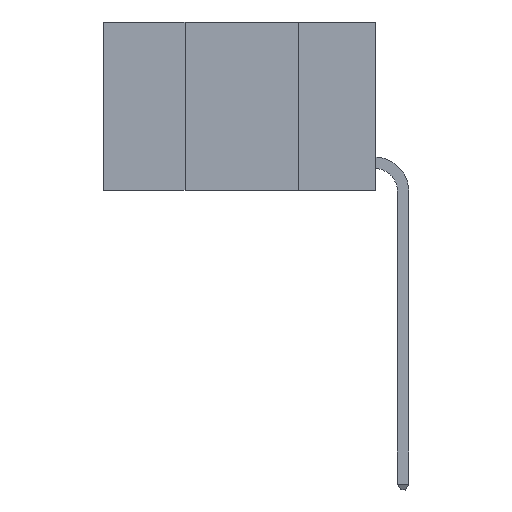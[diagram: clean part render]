
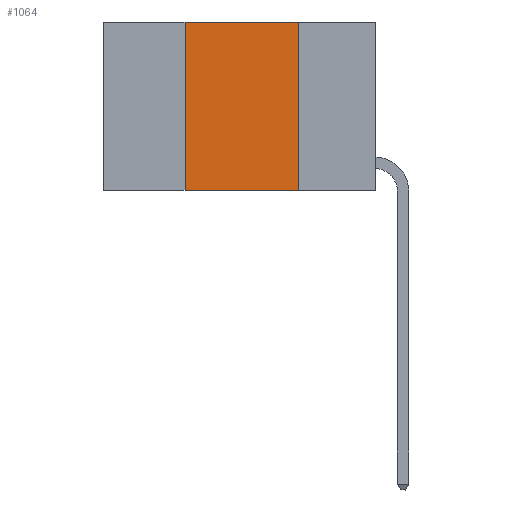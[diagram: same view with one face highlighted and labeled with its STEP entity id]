
A CAD part, left-side view. The second image highlights one B-rep face of the part: STEP entity #1064.
In plain terms, the highlighted planar face has unit normal (-1, 0, 0).
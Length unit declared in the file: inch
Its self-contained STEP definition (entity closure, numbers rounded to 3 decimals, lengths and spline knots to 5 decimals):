
#265 = VERTEX_POINT ( 'NONE', #9439 ) ;
#403 = DIRECTION ( 'NONE',  ( 1., 0., 0. ) ) ;
#446 = LINE ( 'NONE', #10689, #5363 ) ;
#1064 = ADVANCED_FACE ( 'NONE', ( #3475 ), #9762, .F. ) ;
#1499 = EDGE_CURVE ( 'NONE', #8448, #265, #7841, .T. ) ;
#1986 = CARTESIAN_POINT ( 'NONE',  ( 0., 0.42, -0.37 ) ) ;
#2323 = VECTOR ( 'NONE', #11341, 39.37008 ) ;
#2558 = VECTOR ( 'NONE', #10850, 39.37008 ) ;
#2686 = LINE ( 'NONE', #2783, #2323 ) ;
#2783 = CARTESIAN_POINT ( 'NONE',  ( 0., 0.6, 0. ) ) ;
#3475 = FACE_OUTER_BOUND ( 'NONE', #5298, .T. ) ;
#3616 = VECTOR ( 'NONE', #5519, 39.37008 ) ;
#5298 = EDGE_LOOP ( 'NONE', ( #11200, #9071, #10751, #11490 ) ) ;
#5363 = VECTOR ( 'NONE', #6073, 39.37008 ) ;
#5519 = DIRECTION ( 'NONE',  ( 0., 0., 1. ) ) ;
#6073 = DIRECTION ( 'NONE',  ( 0., -1., 0. ) ) ;
#6665 = CARTESIAN_POINT ( 'NONE',  ( 0., 0.42, 0. ) ) ;
#7224 = VERTEX_POINT ( 'NONE', #10201 ) ;
#7841 = LINE ( 'NONE', #6665, #3616 ) ;
#8107 = CARTESIAN_POINT ( 'NONE',  ( 0., 0.17, 0. ) ) ;
#8133 = EDGE_CURVE ( 'NONE', #265, #10884, #2686, .T. ) ;
#8448 = VERTEX_POINT ( 'NONE', #1986 ) ;
#9071 = ORIENTED_EDGE ( 'NONE', *, *, #8133, .F. ) ;
#9258 = EDGE_CURVE ( 'NONE', #8448, #7224, #446, .T. ) ;
#9439 = CARTESIAN_POINT ( 'NONE',  ( 0., 0.42, 0. ) ) ;
#9527 = AXIS2_PLACEMENT_3D ( 'NONE', #12679, #403, #11852 ) ;
#9762 = PLANE ( 'NONE',  #9527 ) ;
#10033 = EDGE_CURVE ( 'NONE', #10884, #7224, #12671, .T. ) ;
#10201 = CARTESIAN_POINT ( 'NONE',  ( 0., 0.17, -0.37 ) ) ;
#10689 = CARTESIAN_POINT ( 'NONE',  ( 0., 0.6, -0.37 ) ) ;
#10751 = ORIENTED_EDGE ( 'NONE', *, *, #1499, .F. ) ;
#10850 = DIRECTION ( 'NONE',  ( 0., 0., -1. ) ) ;
#10884 = VERTEX_POINT ( 'NONE', #10914 ) ;
#10914 = CARTESIAN_POINT ( 'NONE',  ( 0., 0.17, 0. ) ) ;
#11200 = ORIENTED_EDGE ( 'NONE', *, *, #10033, .F. ) ;
#11341 = DIRECTION ( 'NONE',  ( 0., -1., 0. ) ) ;
#11490 = ORIENTED_EDGE ( 'NONE', *, *, #9258, .T. ) ;
#11852 = DIRECTION ( 'NONE',  ( 0., 0., -1. ) ) ;
#12671 = LINE ( 'NONE', #8107, #2558 ) ;
#12679 = CARTESIAN_POINT ( 'NONE',  ( 0., 0.6, 0. ) ) ;
